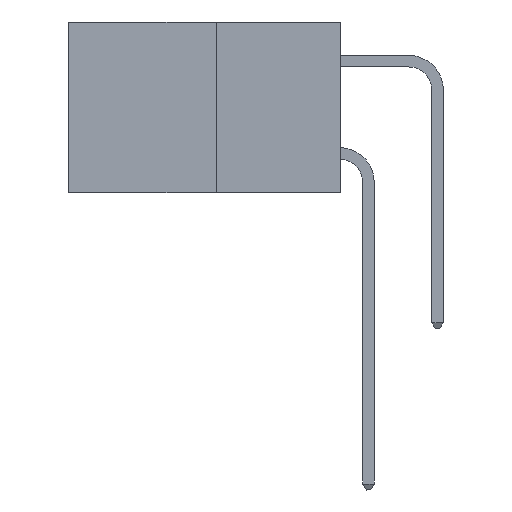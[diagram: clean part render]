
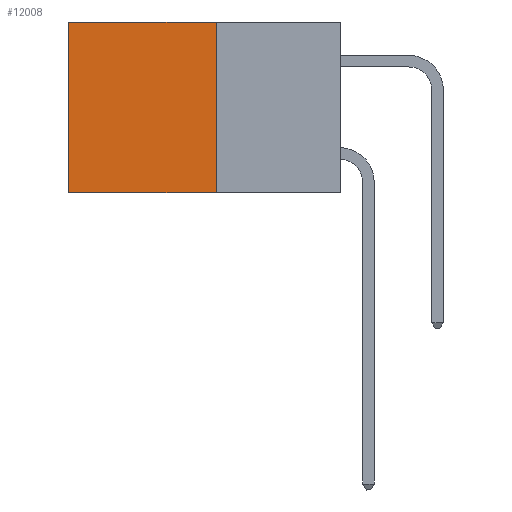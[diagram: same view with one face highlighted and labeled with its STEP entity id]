
A CAD part, left-side view. The second image highlights one B-rep face of the part: STEP entity #12008.
In plain terms, the highlighted planar face has unit normal (-1, 0, 0).
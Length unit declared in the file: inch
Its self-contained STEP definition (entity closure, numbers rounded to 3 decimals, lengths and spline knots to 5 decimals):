
#2427 = EDGE_CURVE ( 'NONE', #29610, #30807, #30435, .T. ) ;
#4147 = EDGE_CURVE ( 'NONE', #21158, #29610, #26817, .T. ) ;
#5509 = EDGE_CURVE ( 'NONE', #21158, #14214, #26713, .T. ) ;
#6035 = LINE ( 'NONE', #16853, #20288 ) ;
#6602 = CARTESIAN_POINT ( 'NONE',  ( 0.277, 0.27, -0.37 ) ) ;
#6726 = DIRECTION ( 'NONE',  ( 0., 0., -1. ) ) ;
#7618 = VECTOR ( 'NONE', #19027, 39.37008 ) ;
#9213 = DIRECTION ( 'NONE',  ( 0., 0., -1. ) ) ;
#11453 = VECTOR ( 'NONE', #35216, 39.37008 ) ;
#12008 = ADVANCED_FACE ( 'NONE', ( #22274 ), #12308, .F. ) ;
#12308 = PLANE ( 'NONE',  #12735 ) ;
#12735 = AXIS2_PLACEMENT_3D ( 'NONE', #6602, #23821, #6726 ) ;
#13296 = CARTESIAN_POINT ( 'NONE',  ( 0.277, 0.27, -0.37 ) ) ;
#14187 = CARTESIAN_POINT ( 'NONE',  ( 0.277, 0.59, -0.37 ) ) ;
#14214 = VERTEX_POINT ( 'NONE', #27836 ) ;
#14236 = CARTESIAN_POINT ( 'NONE',  ( 0.277, 0.27, -0.37 ) ) ;
#14387 = EDGE_LOOP ( 'NONE', ( #26215, #27655, #26546, #14690 ) ) ;
#14690 = ORIENTED_EDGE ( 'NONE', *, *, #5509, .T. ) ;
#16853 = CARTESIAN_POINT ( 'NONE',  ( 0.277, 0.59, -0.37 ) ) ;
#19027 = DIRECTION ( 'NONE',  ( 0., 1., 0. ) ) ;
#19709 = DIRECTION ( 'NONE',  ( 0., 0., -1. ) ) ;
#20288 = VECTOR ( 'NONE', #19709, 39.37008 ) ;
#20577 = CARTESIAN_POINT ( 'NONE',  ( 0.277, 0.27, -0.37 ) ) ;
#21158 = VERTEX_POINT ( 'NONE', #27344 ) ;
#22274 = FACE_OUTER_BOUND ( 'NONE', #14387, .T. ) ;
#23821 = DIRECTION ( 'NONE',  ( 1., 0., 0. ) ) ;
#26215 = ORIENTED_EDGE ( 'NONE', *, *, #27667, .T. ) ;
#26546 = ORIENTED_EDGE ( 'NONE', *, *, #4147, .F. ) ;
#26713 = LINE ( 'NONE', #29506, #11453 ) ;
#26817 = LINE ( 'NONE', #20577, #33483 ) ;
#27344 = CARTESIAN_POINT ( 'NONE',  ( 0.277, 0.27, 0. ) ) ;
#27655 = ORIENTED_EDGE ( 'NONE', *, *, #2427, .F. ) ;
#27667 = EDGE_CURVE ( 'NONE', #14214, #30807, #6035, .T. ) ;
#27836 = CARTESIAN_POINT ( 'NONE',  ( 0.277, 0.59, 0. ) ) ;
#29506 = CARTESIAN_POINT ( 'NONE',  ( 0.277, 0.27, 0. ) ) ;
#29610 = VERTEX_POINT ( 'NONE', #14236 ) ;
#30435 = LINE ( 'NONE', #13296, #7618 ) ;
#30807 = VERTEX_POINT ( 'NONE', #14187 ) ;
#33483 = VECTOR ( 'NONE', #9213, 39.37008 ) ;
#35216 = DIRECTION ( 'NONE',  ( 0., 1., 0. ) ) ;
